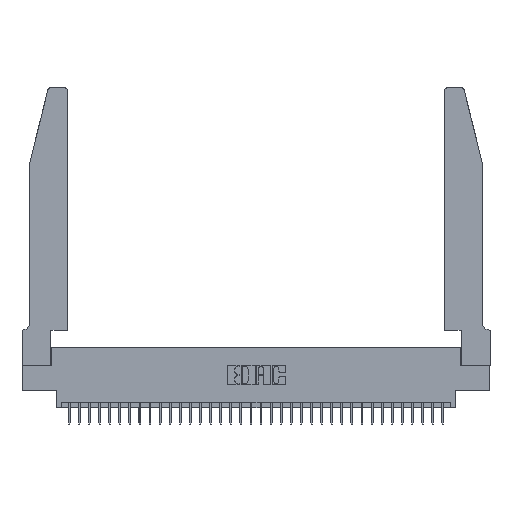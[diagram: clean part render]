
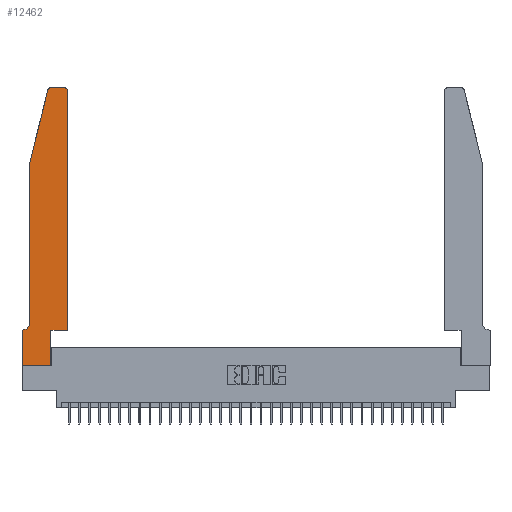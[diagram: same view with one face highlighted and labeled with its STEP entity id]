
A CAD part, top view. The second image highlights one B-rep face of the part: STEP entity #12462.
In plain terms, the highlighted planar face has unit normal (0, 0, 1).
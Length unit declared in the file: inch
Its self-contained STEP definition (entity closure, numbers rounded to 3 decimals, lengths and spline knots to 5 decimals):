
#782 = VERTEX_POINT ( 'NONE', #11619 ) ;
#885 = DIRECTION ( 'NONE',  ( 0., 0., 1. ) ) ;
#1003 = AXIS2_PLACEMENT_3D ( 'NONE', #11231, #30312, #14016 ) ;
#2795 = EDGE_CURVE ( 'NONE', #7184, #19175, #24034, .T. ) ;
#3329 = CARTESIAN_POINT ( 'NONE',  ( 0.4205, 2.75, 0.37 ) ) ;
#3585 = LINE ( 'NONE', #33949, #11802 ) ;
#4330 = CARTESIAN_POINT ( 'NONE',  ( 0.0755, 2., 0.37 ) ) ;
#4423 = CARTESIAN_POINT ( 'NONE',  ( 0.25487, 2.72718, 0.37 ) ) ;
#4586 = CIRCLE ( 'NONE', #1003, 0.03 ) ;
#4587 = ORIENTED_EDGE ( 'NONE', *, *, #6000, .T. ) ;
#4755 = LINE ( 'NONE', #5551, #11252 ) ;
#4763 = VERTEX_POINT ( 'NONE', #30990 ) ;
#4905 = VERTEX_POINT ( 'NONE', #26244 ) ;
#5551 = CARTESIAN_POINT ( 'NONE',  ( 0.2865, 0.35, 0.37 ) ) ;
#5998 = EDGE_CURVE ( 'NONE', #19175, #27593, #32663, .T. ) ;
#6000 = EDGE_CURVE ( 'NONE', #4763, #4905, #3585, .T. ) ;
#6693 = EDGE_CURVE ( 'NONE', #782, #13836, #33896, .T. ) ;
#7021 = CARTESIAN_POINT ( 'NONE',  ( 0.0755, 0.35, 0.37 ) ) ;
#7184 = VERTEX_POINT ( 'NONE', #21653 ) ;
#7188 = EDGE_CURVE ( 'NONE', #34836, #4763, #33008, .T. ) ;
#7782 = ORIENTED_EDGE ( 'NONE', *, *, #6693, .T. ) ;
#7891 = CARTESIAN_POINT ( 'NONE',  ( 0.2605, 2.75, 0.37 ) ) ;
#7940 = ORIENTED_EDGE ( 'NONE', *, *, #9261, .T. ) ;
#8273 = EDGE_LOOP ( 'NONE', ( #22469, #8990, #21242, #7940, #7782, #19518, #30860, #4587, #12720, #9817, #10199, #33868 ) ) ;
#8346 = DIRECTION ( 'NONE',  ( 0., 1., 0. ) ) ;
#8627 = PLANE ( 'NONE',  #30223 ) ;
#8664 = VECTOR ( 'NONE', #26229, 39.37008 ) ;
#8942 = DIRECTION ( 'NONE',  ( 1., 0., 0. ) ) ;
#8990 = ORIENTED_EDGE ( 'NONE', *, *, #22789, .T. ) ;
#9261 = EDGE_CURVE ( 'NONE', #27423, #782, #30619, .T. ) ;
#9357 = CARTESIAN_POINT ( 'NONE',  ( 0.0055, 0.42, 0.37 ) ) ;
#9817 = ORIENTED_EDGE ( 'NONE', *, *, #2795, .T. ) ;
#10199 = ORIENTED_EDGE ( 'NONE', *, *, #5998, .T. ) ;
#10714 = DIRECTION ( 'NONE',  ( 0., -1., 0. ) ) ;
#11231 = CARTESIAN_POINT ( 'NONE',  ( 0.4205, 2.72, 0.37 ) ) ;
#11252 = VECTOR ( 'NONE', #8346, 39.37008 ) ;
#11619 = CARTESIAN_POINT ( 'NONE',  ( 0.0755, 0.42, 0.37 ) ) ;
#11802 = VECTOR ( 'NONE', #17762, 39.37008 ) ;
#12072 = CARTESIAN_POINT ( 'NONE',  ( 0.4505, 0.35, 0.37 ) ) ;
#12151 = DIRECTION ( 'NONE',  ( -1., 0., 0. ) ) ;
#12394 = VECTOR ( 'NONE', #21612, 39.37008 ) ;
#12462 = ADVANCED_FACE ( 'NONE', ( #31697 ), #8627, .T. ) ;
#12720 = ORIENTED_EDGE ( 'NONE', *, *, #22570, .T. ) ;
#13266 = LINE ( 'NONE', #7891, #12394 ) ;
#13413 = CIRCLE ( 'NONE', #19057, 0.03 ) ;
#13836 = VERTEX_POINT ( 'NONE', #28073 ) ;
#14016 = DIRECTION ( 'NONE',  ( 1., 0., 0. ) ) ;
#14339 = DIRECTION ( 'NONE',  ( 1., 0., 0. ) ) ;
#14398 = AXIS2_PLACEMENT_3D ( 'NONE', #9357, #28467, #12151 ) ;
#15323 = VECTOR ( 'NONE', #30651, 39.37008 ) ;
#16188 = CARTESIAN_POINT ( 'NONE',  ( 0., 0., 0.37 ) ) ;
#16524 = CARTESIAN_POINT ( 'NONE',  ( 0.0755, 2., 0.37 ) ) ;
#16817 = VECTOR ( 'NONE', #8942, 39.37008 ) ;
#17389 = EDGE_CURVE ( 'NONE', #18959, #27423, #20809, .T. ) ;
#17433 = CARTESIAN_POINT ( 'NONE',  ( 0.284, 2.72, 0.37 ) ) ;
#17762 = DIRECTION ( 'NONE',  ( 1., 0., 0. ) ) ;
#18919 = CARTESIAN_POINT ( 'NONE',  ( 0.4505, 2.72, 0.37 ) ) ;
#18959 = VERTEX_POINT ( 'NONE', #4423 ) ;
#19057 = AXIS2_PLACEMENT_3D ( 'NONE', #17433, #885, #20135 ) ;
#19175 = VERTEX_POINT ( 'NONE', #25066 ) ;
#19518 = ORIENTED_EDGE ( 'NONE', *, *, #28646, .T. ) ;
#19905 = CARTESIAN_POINT ( 'NONE',  ( 0.4505, 0.35, 0.37 ) ) ;
#20135 = DIRECTION ( 'NONE',  ( 1., 0., 0. ) ) ;
#20385 = EDGE_CURVE ( 'NONE', #27593, #35020, #4586, .T. ) ;
#20579 = VERTEX_POINT ( 'NONE', #33724 ) ;
#20809 = LINE ( 'NONE', #16524, #26332 ) ;
#21242 = ORIENTED_EDGE ( 'NONE', *, *, #17389, .T. ) ;
#21612 = DIRECTION ( 'NONE',  ( -1., 0., 0. ) ) ;
#21652 = CARTESIAN_POINT ( 'NONE',  ( 0., 0.35, 0.37 ) ) ;
#21653 = CARTESIAN_POINT ( 'NONE',  ( 0.2865, 0.35, 0.37 ) ) ;
#22437 = LINE ( 'NONE', #7021, #8664 ) ;
#22469 = ORIENTED_EDGE ( 'NONE', *, *, #30800, .T. ) ;
#22570 = EDGE_CURVE ( 'NONE', #4905, #7184, #4755, .T. ) ;
#22789 = EDGE_CURVE ( 'NONE', #20579, #18959, #13413, .T. ) ;
#23101 = DIRECTION ( 'NONE',  ( 0., 1., 0. ) ) ;
#24034 = LINE ( 'NONE', #19905, #16817 ) ;
#25066 = CARTESIAN_POINT ( 'NONE',  ( 0.4505, 0.35, 0.37 ) ) ;
#25504 = VECTOR ( 'NONE', #23101, 39.37008 ) ;
#25844 = VECTOR ( 'NONE', #10714, 39.37008 ) ;
#26229 = DIRECTION ( 'NONE',  ( -1., 0., 0. ) ) ;
#26244 = CARTESIAN_POINT ( 'NONE',  ( 0.2865, 0., 0.37 ) ) ;
#26332 = VECTOR ( 'NONE', #32843, 39.37008 ) ;
#27423 = VERTEX_POINT ( 'NONE', #4330 ) ;
#27593 = VERTEX_POINT ( 'NONE', #18919 ) ;
#27888 = CARTESIAN_POINT ( 'NONE',  ( 0., 0.35, 0.37 ) ) ;
#27911 = CARTESIAN_POINT ( 'NONE',  ( 0.0755, 2., 0.37 ) ) ;
#28073 = CARTESIAN_POINT ( 'NONE',  ( 0.0055, 0.35, 0.37 ) ) ;
#28467 = DIRECTION ( 'NONE',  ( 0., 0., -1. ) ) ;
#28646 = EDGE_CURVE ( 'NONE', #13836, #34836, #22437, .T. ) ;
#30223 = AXIS2_PLACEMENT_3D ( 'NONE', #27888, #30629, #14339 ) ;
#30312 = DIRECTION ( 'NONE',  ( 0., 0., 1. ) ) ;
#30619 = LINE ( 'NONE', #27911, #15323 ) ;
#30629 = DIRECTION ( 'NONE',  ( 0., 0., 1. ) ) ;
#30651 = DIRECTION ( 'NONE',  ( 0., -1., 0. ) ) ;
#30800 = EDGE_CURVE ( 'NONE', #35020, #20579, #13266, .T. ) ;
#30860 = ORIENTED_EDGE ( 'NONE', *, *, #7188, .T. ) ;
#30990 = CARTESIAN_POINT ( 'NONE',  ( 0., 0., 0.37 ) ) ;
#31697 = FACE_OUTER_BOUND ( 'NONE', #8273, .T. ) ;
#32663 = LINE ( 'NONE', #12072, #25504 ) ;
#32843 = DIRECTION ( 'NONE',  ( -0.239, -0.971, 0. ) ) ;
#33008 = LINE ( 'NONE', #16188, #25844 ) ;
#33724 = CARTESIAN_POINT ( 'NONE',  ( 0.284, 2.75, 0.37 ) ) ;
#33868 = ORIENTED_EDGE ( 'NONE', *, *, #20385, .T. ) ;
#33896 = CIRCLE ( 'NONE', #14398, 0.07 ) ;
#33949 = CARTESIAN_POINT ( 'NONE',  ( 0., 0., 0.37 ) ) ;
#34836 = VERTEX_POINT ( 'NONE', #21652 ) ;
#35020 = VERTEX_POINT ( 'NONE', #3329 ) ;
